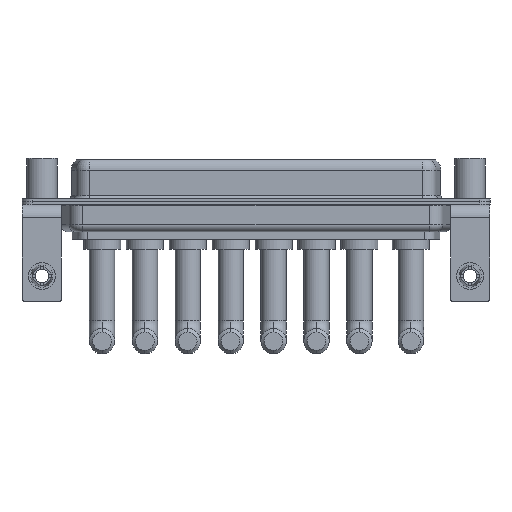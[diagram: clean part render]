
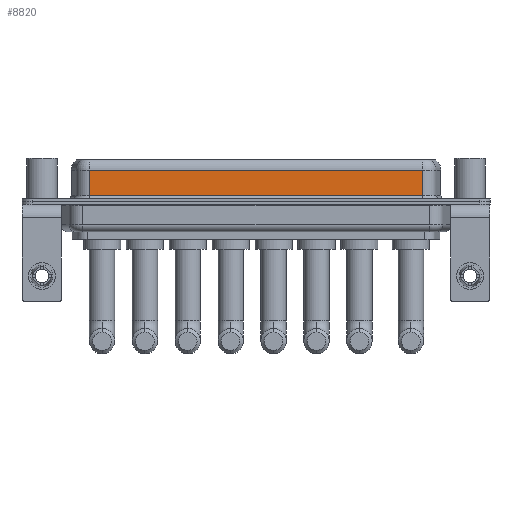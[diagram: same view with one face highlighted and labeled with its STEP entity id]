
A CAD part, front view. The second image highlights one B-rep face of the part: STEP entity #8820.
In plain terms, the highlighted planar face has unit normal (0, -1, 0).
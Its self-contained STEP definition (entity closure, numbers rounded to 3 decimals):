
#158 = LINE ( 'NONE', #10285, #2506 ) ;
#1106 = DIRECTION ( 'NONE',  ( 0., 0., -1. ) ) ;
#1326 = LINE ( 'NONE', #6522, #13078 ) ;
#1367 = EDGE_LOOP ( 'NONE', ( #14292, #14433, #15850, #11479 ) ) ;
#2015 = DIRECTION ( 'NONE',  ( 1., 0., 0. ) ) ;
#2470 = CARTESIAN_POINT ( 'NONE',  ( 7.038, -3.95, 6.4 ) ) ;
#2506 = VECTOR ( 'NONE', #14194, 1000. ) ;
#2824 = VERTEX_POINT ( 'NONE', #15580 ) ;
#3080 = VECTOR ( 'NONE', #1106, 1000. ) ;
#3790 = VECTOR ( 'NONE', #2015, 1000. ) ;
#4013 = PLANE ( 'NONE',  #13363 ) ;
#4650 = CARTESIAN_POINT ( 'NONE',  ( 56.462, -3.95, 0.9 ) ) ;
#5978 = VERTEX_POINT ( 'NONE', #11657 ) ;
#6228 = EDGE_CURVE ( 'NONE', #10250, #2824, #16566, .T. ) ;
#6500 = FACE_OUTER_BOUND ( 'NONE', #1367, .T. ) ;
#6522 = CARTESIAN_POINT ( 'NONE',  ( 56.462, -3.95, 4.65 ) ) ;
#8365 = EDGE_CURVE ( 'NONE', #5978, #16156, #1326, .T. ) ;
#8820 = ADVANCED_FACE ( 'NONE', ( #6500 ), #4013, .F. ) ;
#9214 = DIRECTION ( 'NONE',  ( 0., 1., 0. ) ) ;
#10130 = EDGE_CURVE ( 'NONE', #16156, #10250, #14281, .T. ) ;
#10158 = EDGE_CURVE ( 'NONE', #5978, #2824, #158, .T. ) ;
#10250 = VERTEX_POINT ( 'NONE', #16220 ) ;
#10285 = CARTESIAN_POINT ( 'NONE',  ( 56.462, -3.95, 6.4 ) ) ;
#11479 = ORIENTED_EDGE ( 'NONE', *, *, #6228, .T. ) ;
#11657 = CARTESIAN_POINT ( 'NONE',  ( 56.462, -3.95, 4.65 ) ) ;
#11664 = DIRECTION ( 'NONE',  ( 0., 0., 1. ) ) ;
#11778 = DIRECTION ( 'NONE',  ( -1., 0., 0. ) ) ;
#12133 = CARTESIAN_POINT ( 'NONE',  ( 7.038, -3.95, 4.65 ) ) ;
#12955 = CARTESIAN_POINT ( 'NONE',  ( 56.462, -3.95, 6.4 ) ) ;
#13078 = VECTOR ( 'NONE', #11778, 1000. ) ;
#13363 = AXIS2_PLACEMENT_3D ( 'NONE', #12955, #9214, #11664 ) ;
#14194 = DIRECTION ( 'NONE',  ( 0., 0., -1. ) ) ;
#14281 = LINE ( 'NONE', #2470, #3080 ) ;
#14292 = ORIENTED_EDGE ( 'NONE', *, *, #10158, .F. ) ;
#14433 = ORIENTED_EDGE ( 'NONE', *, *, #8365, .T. ) ;
#15580 = CARTESIAN_POINT ( 'NONE',  ( 56.462, -3.95, 0.9 ) ) ;
#15850 = ORIENTED_EDGE ( 'NONE', *, *, #10130, .T. ) ;
#16156 = VERTEX_POINT ( 'NONE', #12133 ) ;
#16220 = CARTESIAN_POINT ( 'NONE',  ( 7.038, -3.95, 0.9 ) ) ;
#16566 = LINE ( 'NONE', #4650, #3790 ) ;
